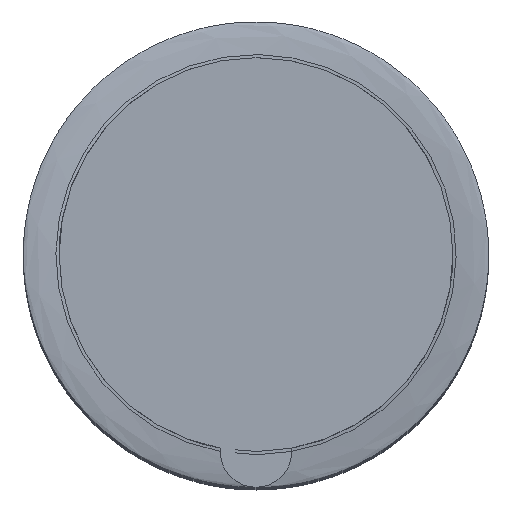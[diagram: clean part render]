
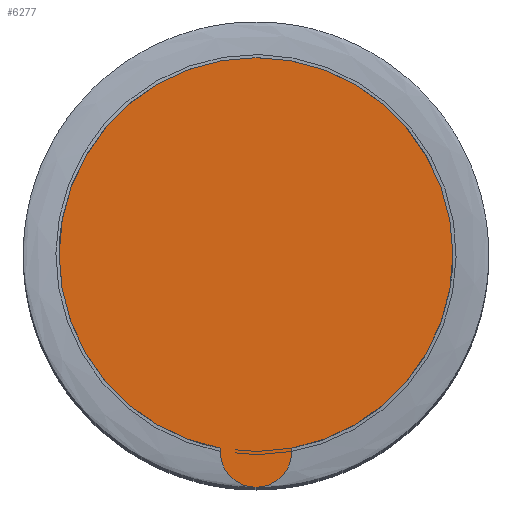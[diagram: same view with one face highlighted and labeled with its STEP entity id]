
A CAD part, top view. The second image highlights one B-rep face of the part: STEP entity #6277.
In plain terms, the highlighted planar face has unit normal (0, 0, 1).
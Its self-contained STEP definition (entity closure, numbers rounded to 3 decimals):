
#99 = AXIS2_PLACEMENT_3D ( 'NONE', #3001, #6652, #3521 ) ;
#247 = ORIENTED_EDGE ( 'NONE', *, *, #4555, .T. ) ;
#398 = DIRECTION ( 'NONE',  ( 0., 0., 1. ) ) ;
#472 = AXIS2_PLACEMENT_3D ( 'NONE', #6136, #398, #4057 ) ;
#536 = DIRECTION ( 'NONE',  ( 0., 0., 1. ) ) ;
#723 = DIRECTION ( 'NONE',  ( 0., 0., 1. ) ) ;
#737 = CARTESIAN_POINT ( 'NONE',  ( -5., 23.292, 23. ) ) ;
#787 = DIRECTION ( 'NONE',  ( 1., 0., 0. ) ) ;
#806 = DIRECTION ( 'NONE',  ( 0., 0., 1. ) ) ;
#858 = CIRCLE ( 'NONE', #2633, 0.5 ) ;
#890 = CARTESIAN_POINT ( 'NONE',  ( -5., 23.292, 23. ) ) ;
#935 = EDGE_CURVE ( 'NONE', #3997, #2286, #1271, .T. ) ;
#1087 = CARTESIAN_POINT ( 'NONE',  ( -5.498, 20.588, 23. ) ) ;
#1264 = DIRECTION ( 'NONE',  ( 1., 0., 0. ) ) ;
#1271 = CIRCLE ( 'NONE', #6610, 2.75 ) ;
#1477 = AXIS2_PLACEMENT_3D ( 'NONE', #3871, #723, #4390 ) ;
#1541 = ORIENTED_EDGE ( 'NONE', *, *, #935, .T. ) ;
#1834 = CARTESIAN_POINT ( 'NONE',  ( -7.75, 23.292, 23. ) ) ;
#1878 = PLANE ( 'NONE',  #472 ) ;
#1913 = CIRCLE ( 'NONE', #2262, 0.5 ) ;
#2078 = DIRECTION ( 'NONE',  ( 0., 0., 1. ) ) ;
#2262 = AXIS2_PLACEMENT_3D ( 'NONE', #3673, #536, #4200 ) ;
#2286 = VERTEX_POINT ( 'NONE', #1087 ) ;
#2633 = AXIS2_PLACEMENT_3D ( 'NONE', #5224, #2078, #5748 ) ;
#2694 = VERTEX_POINT ( 'NONE', #2823 ) ;
#2738 = EDGE_CURVE ( 'NONE', #2875, #6463, #4476, .T. ) ;
#2823 = CARTESIAN_POINT ( 'NONE',  ( -5.5, 20.542, 23. ) ) ;
#2875 = VERTEX_POINT ( 'NONE', #5950 ) ;
#2980 = CARTESIAN_POINT ( 'NONE',  ( -2.25, 23.292, 23. ) ) ;
#3001 = CARTESIAN_POINT ( 'NONE',  ( -5., 20.542, 23. ) ) ;
#3521 = DIRECTION ( 'NONE',  ( 1., 0., 0. ) ) ;
#3558 = CIRCLE ( 'NONE', #1477, 2.75 ) ;
#3592 = AXIS2_PLACEMENT_3D ( 'NONE', #737, #4402, #1264 ) ;
#3673 = CARTESIAN_POINT ( 'NONE',  ( -5., 20.542, 23. ) ) ;
#3871 = CARTESIAN_POINT ( 'NONE',  ( -5., 23.292, 23. ) ) ;
#3974 = CIRCLE ( 'NONE', #99, 0.5 ) ;
#3997 = VERTEX_POINT ( 'NONE', #1834 ) ;
#4057 = DIRECTION ( 'NONE',  ( 1., 0., 0. ) ) ;
#4071 = ORIENTED_EDGE ( 'NONE', *, *, #6631, .T. ) ;
#4200 = DIRECTION ( 'NONE',  ( 1., 0., 0. ) ) ;
#4312 = FACE_OUTER_BOUND ( 'NONE', #4920, .T. ) ;
#4390 = DIRECTION ( 'NONE',  ( 1., 0., 0. ) ) ;
#4402 = DIRECTION ( 'NONE',  ( 0., 0., 1. ) ) ;
#4476 = CIRCLE ( 'NONE', #3592, 2.75 ) ;
#4496 = EDGE_CURVE ( 'NONE', #6100, #2875, #858, .T. ) ;
#4555 = EDGE_CURVE ( 'NONE', #2286, #2694, #1913, .T. ) ;
#4760 = ORIENTED_EDGE ( 'NONE', *, *, #5600, .T. ) ;
#4920 = EDGE_LOOP ( 'NONE', ( #5962, #4760, #1541, #247, #4071, #6547 ) ) ;
#5023 = CARTESIAN_POINT ( 'NONE',  ( -4.5, 20.542, 23. ) ) ;
#5224 = CARTESIAN_POINT ( 'NONE',  ( -5., 20.542, 23. ) ) ;
#5600 = EDGE_CURVE ( 'NONE', #6463, #3997, #3558, .T. ) ;
#5748 = DIRECTION ( 'NONE',  ( 1., 0., 0. ) ) ;
#5950 = CARTESIAN_POINT ( 'NONE',  ( -4.502, 20.588, 23. ) ) ;
#5962 = ORIENTED_EDGE ( 'NONE', *, *, #2738, .T. ) ;
#6100 = VERTEX_POINT ( 'NONE', #5023 ) ;
#6136 = CARTESIAN_POINT ( 'NONE',  ( -5., 23.292, 23. ) ) ;
#6277 = ADVANCED_FACE ( 'NONE', ( #4312 ), #1878, .T. ) ;
#6463 = VERTEX_POINT ( 'NONE', #2980 ) ;
#6547 = ORIENTED_EDGE ( 'NONE', *, *, #4496, .T. ) ;
#6610 = AXIS2_PLACEMENT_3D ( 'NONE', #890, #806, #787 ) ;
#6631 = EDGE_CURVE ( 'NONE', #2694, #6100, #3974, .T. ) ;
#6652 = DIRECTION ( 'NONE',  ( 0., 0., 1. ) ) ;
